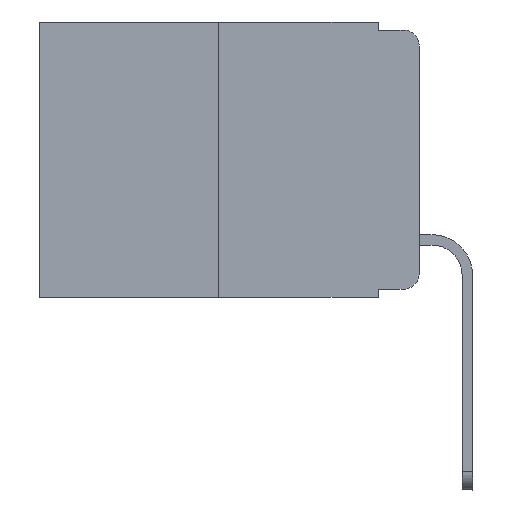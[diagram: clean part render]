
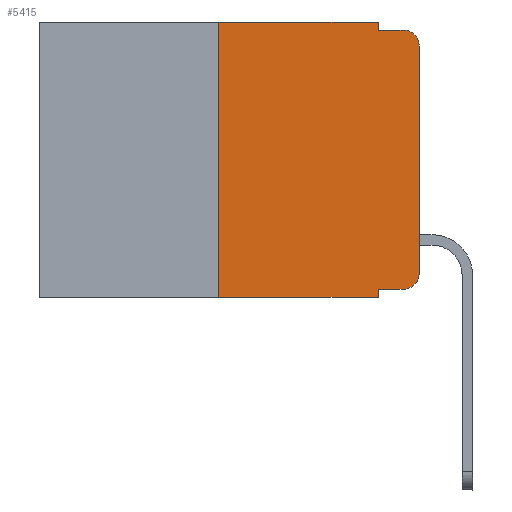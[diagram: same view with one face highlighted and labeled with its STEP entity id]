
A CAD part, left-side view. The second image highlights one B-rep face of the part: STEP entity #5415.
In plain terms, the highlighted planar face has unit normal (-1, 0, 0).
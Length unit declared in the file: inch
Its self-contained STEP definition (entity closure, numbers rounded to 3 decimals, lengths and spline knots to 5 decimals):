
#62 = ORIENTED_EDGE ( 'NONE', *, *, #623, .F. ) ;
#134 = EDGE_CURVE ( 'NONE', #2539, #7770, #6196, .T. ) ;
#226 = ORIENTED_EDGE ( 'NONE', *, *, #594, .T. ) ;
#362 = DIRECTION ( 'NONE',  ( 0., -1., 0. ) ) ;
#394 = DIRECTION ( 'NONE',  ( -1., 0., 0. ) ) ;
#571 = CARTESIAN_POINT ( 'NONE',  ( 0., 0.473, 0. ) ) ;
#592 = ORIENTED_EDGE ( 'NONE', *, *, #1629, .F. ) ;
#594 = EDGE_CURVE ( 'NONE', #864, #2593, #7817, .T. ) ;
#600 = DIRECTION ( 'NONE',  ( 0., 0., -1. ) ) ;
#623 = EDGE_CURVE ( 'NONE', #9051, #6749, #2165, .T. ) ;
#663 = FACE_OUTER_BOUND ( 'NONE', #9198, .T. ) ;
#673 = ORIENTED_EDGE ( 'NONE', *, *, #3161, .T. ) ;
#864 = VERTEX_POINT ( 'NONE', #3322 ) ;
#1003 = CARTESIAN_POINT ( 'NONE',  ( 0., 0.02, -0.03 ) ) ;
#1254 = LINE ( 'NONE', #571, #7125 ) ;
#1507 = DIRECTION ( 'NONE',  ( 0., 0., -1. ) ) ;
#1521 = ORIENTED_EDGE ( 'NONE', *, *, #5197, .T. ) ;
#1629 = EDGE_CURVE ( 'NONE', #6898, #3831, #4024, .T. ) ;
#2158 = VECTOR ( 'NONE', #2853, 39.37008 ) ;
#2165 = LINE ( 'NONE', #2852, #7082 ) ;
#2393 = AXIS2_PLACEMENT_3D ( 'NONE', #1003, #3571, #4152 ) ;
#2507 = EDGE_CURVE ( 'NONE', #2539, #8905, #8703, .T. ) ;
#2539 = VERTEX_POINT ( 'NONE', #9647 ) ;
#2591 = AXIS2_PLACEMENT_3D ( 'NONE', #10309, #3065, #1507 ) ;
#2593 = VERTEX_POINT ( 'NONE', #4150 ) ;
#2672 = CARTESIAN_POINT ( 'NONE',  ( 0., 0.25, 0. ) ) ;
#2678 = CARTESIAN_POINT ( 'NONE',  ( 0., 0.051, -0.01 ) ) ;
#2771 = EDGE_CURVE ( 'NONE', #3831, #9051, #1254, .T. ) ;
#2852 = CARTESIAN_POINT ( 'NONE',  ( 0., 0.051, 0. ) ) ;
#2853 = DIRECTION ( 'NONE',  ( 0., 0., -1. ) ) ;
#3065 = DIRECTION ( 'NONE',  ( 1., 0., 0. ) ) ;
#3081 = CARTESIAN_POINT ( 'NONE',  ( 0., 0.051, -0.01 ) ) ;
#3161 = EDGE_CURVE ( 'NONE', #6898, #7770, #6781, .T. ) ;
#3202 = CARTESIAN_POINT ( 'NONE',  ( 0., 0.051, -0.333 ) ) ;
#3249 = CIRCLE ( 'NONE', #3760, 0.02 ) ;
#3286 = CARTESIAN_POINT ( 'NONE',  ( 0., 0.02, -0.333 ) ) ;
#3322 = CARTESIAN_POINT ( 'NONE',  ( 0., 0., -0.313 ) ) ;
#3562 = VECTOR ( 'NONE', #8996, 39.37008 ) ;
#3571 = DIRECTION ( 'NONE',  ( -1., 0., 0. ) ) ;
#3574 = VECTOR ( 'NONE', #9588, 39.37008 ) ;
#3760 = AXIS2_PLACEMENT_3D ( 'NONE', #5281, #394, #6879 ) ;
#3796 = EDGE_CURVE ( 'NONE', #2593, #7479, #5422, .T. ) ;
#3831 = VERTEX_POINT ( 'NONE', #2672 ) ;
#3864 = PLANE ( 'NONE',  #2591 ) ;
#3967 = CARTESIAN_POINT ( 'NONE',  ( 0., 0.051, 0. ) ) ;
#4024 = LINE ( 'NONE', #9674, #3562 ) ;
#4150 = CARTESIAN_POINT ( 'NONE',  ( 0., 0., -0.03 ) ) ;
#4152 = DIRECTION ( 'NONE',  ( 0., 0., -1. ) ) ;
#4912 = EDGE_CURVE ( 'NONE', #6749, #7479, #5853, .T. ) ;
#4970 = ORIENTED_EDGE ( 'NONE', *, *, #2771, .F. ) ;
#5049 = VECTOR ( 'NONE', #9242, 39.37008 ) ;
#5197 = EDGE_CURVE ( 'NONE', #8905, #864, #3249, .T. ) ;
#5281 = CARTESIAN_POINT ( 'NONE',  ( 0., 0.02, -0.313 ) ) ;
#5388 = CARTESIAN_POINT ( 'NONE',  ( 0., 0.051, 0. ) ) ;
#5415 = ADVANCED_FACE ( 'NONE', ( #663 ), #3864, .F. ) ;
#5422 = CIRCLE ( 'NONE', #2393, 0.02 ) ;
#5843 = CARTESIAN_POINT ( 'NONE',  ( 0., 0.051, -0.343 ) ) ;
#5853 = LINE ( 'NONE', #2678, #7638 ) ;
#5911 = ORIENTED_EDGE ( 'NONE', *, *, #4912, .F. ) ;
#6028 = CARTESIAN_POINT ( 'NONE',  ( 0., 0., 0. ) ) ;
#6196 = LINE ( 'NONE', #5388, #2158 ) ;
#6749 = VERTEX_POINT ( 'NONE', #3081 ) ;
#6781 = LINE ( 'NONE', #10046, #8611 ) ;
#6879 = DIRECTION ( 'NONE',  ( 0., 0., -1. ) ) ;
#6898 = VERTEX_POINT ( 'NONE', #8149 ) ;
#7082 = VECTOR ( 'NONE', #600, 39.37008 ) ;
#7125 = VECTOR ( 'NONE', #9312, 39.37008 ) ;
#7415 = ORIENTED_EDGE ( 'NONE', *, *, #134, .F. ) ;
#7479 = VERTEX_POINT ( 'NONE', #9379 ) ;
#7571 = DIRECTION ( 'NONE',  ( 0., -1., 0. ) ) ;
#7638 = VECTOR ( 'NONE', #362, 39.37008 ) ;
#7770 = VERTEX_POINT ( 'NONE', #5843 ) ;
#7817 = LINE ( 'NONE', #6028, #5049 ) ;
#8149 = CARTESIAN_POINT ( 'NONE',  ( 0., 0.25, -0.343 ) ) ;
#8502 = ORIENTED_EDGE ( 'NONE', *, *, #2507, .T. ) ;
#8611 = VECTOR ( 'NONE', #7571, 39.37008 ) ;
#8703 = LINE ( 'NONE', #3202, #3574 ) ;
#8905 = VERTEX_POINT ( 'NONE', #3286 ) ;
#8996 = DIRECTION ( 'NONE',  ( 0., 0., 1. ) ) ;
#9051 = VERTEX_POINT ( 'NONE', #3967 ) ;
#9198 = EDGE_LOOP ( 'NONE', ( #226, #9411, #5911, #62, #4970, #592, #673, #7415, #8502, #1521 ) ) ;
#9242 = DIRECTION ( 'NONE',  ( 0., 0., 1. ) ) ;
#9312 = DIRECTION ( 'NONE',  ( 0., -1., 0. ) ) ;
#9379 = CARTESIAN_POINT ( 'NONE',  ( 0., 0.02, -0.01 ) ) ;
#9411 = ORIENTED_EDGE ( 'NONE', *, *, #3796, .T. ) ;
#9588 = DIRECTION ( 'NONE',  ( 0., -1., 0. ) ) ;
#9647 = CARTESIAN_POINT ( 'NONE',  ( 0., 0.051, -0.333 ) ) ;
#9674 = CARTESIAN_POINT ( 'NONE',  ( 0., 0.25, 0. ) ) ;
#10046 = CARTESIAN_POINT ( 'NONE',  ( 0., 0.473, -0.343 ) ) ;
#10309 = CARTESIAN_POINT ( 'NONE',  ( 0., 0.473, 0. ) ) ;
